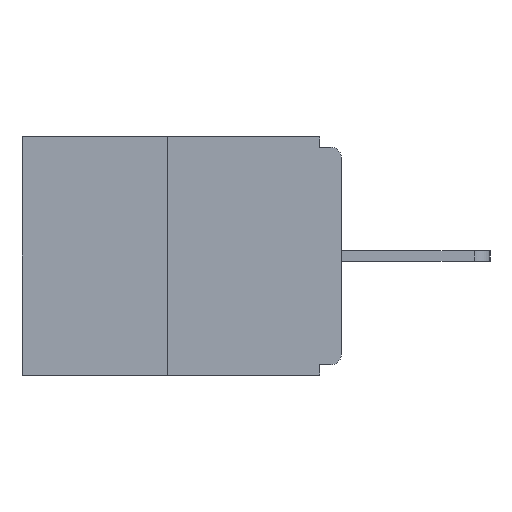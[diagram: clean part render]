
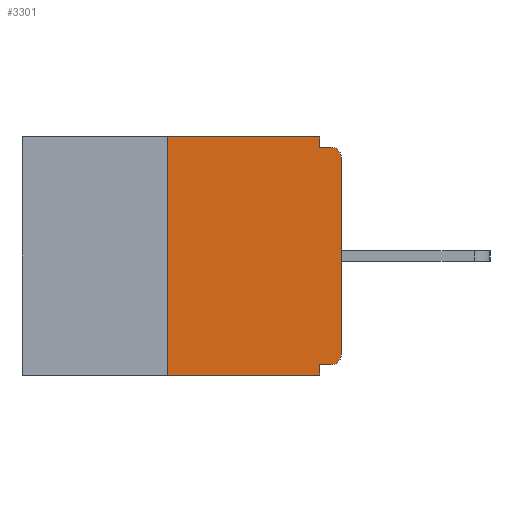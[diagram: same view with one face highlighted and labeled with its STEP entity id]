
A CAD part, left-side view. The second image highlights one B-rep face of the part: STEP entity #3301.
In plain terms, the highlighted planar face has unit normal (-1, 0, 0).
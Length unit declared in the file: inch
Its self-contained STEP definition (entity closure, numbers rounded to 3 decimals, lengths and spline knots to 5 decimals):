
#242 = CARTESIAN_POINT ( 'NONE',  ( 0., 0.031, -0.343 ) ) ;
#343 = CARTESIAN_POINT ( 'NONE',  ( 0., 0., -0.03 ) ) ;
#456 = VERTEX_POINT ( 'NONE', #1524 ) ;
#548 = VECTOR ( 'NONE', #8571, 39.37008 ) ;
#653 = DIRECTION ( 'NONE',  ( -1., 0., 0. ) ) ;
#758 = DIRECTION ( 'NONE',  ( -1., 0., 0. ) ) ;
#955 = LINE ( 'NONE', #3076, #10718 ) ;
#1160 = LINE ( 'NONE', #10264, #548 ) ;
#1182 = AXIS2_PLACEMENT_3D ( 'NONE', #12285, #2567, #3556 ) ;
#1368 = LINE ( 'NONE', #5953, #6409 ) ;
#1451 = CARTESIAN_POINT ( 'NONE',  ( 0., 0.46, -0.343 ) ) ;
#1524 = CARTESIAN_POINT ( 'NONE',  ( 0., 0.031, -0.328 ) ) ;
#1727 = DIRECTION ( 'NONE',  ( 0., 0., -1. ) ) ;
#2088 = VECTOR ( 'NONE', #8111, 39.37008 ) ;
#2567 = DIRECTION ( 'NONE',  ( 1., 0., 0. ) ) ;
#2926 = VECTOR ( 'NONE', #6526, 39.37008 ) ;
#3076 = CARTESIAN_POINT ( 'NONE',  ( 0., 0., -0.015 ) ) ;
#3214 = VERTEX_POINT ( 'NONE', #10161 ) ;
#3280 = EDGE_CURVE ( 'NONE', #8709, #8806, #3807, .T. ) ;
#3301 = ADVANCED_FACE ( 'NONE', ( #7441 ), #3514, .F. ) ;
#3380 = CARTESIAN_POINT ( 'NONE',  ( 0., 0.015, -0.015 ) ) ;
#3514 = PLANE ( 'NONE',  #1182 ) ;
#3556 = DIRECTION ( 'NONE',  ( 0., 0., -1. ) ) ;
#3696 = EDGE_CURVE ( 'NONE', #6570, #8709, #9564, .T. ) ;
#3751 = DIRECTION ( 'NONE',  ( 0., 0., 1. ) ) ;
#3774 = ORIENTED_EDGE ( 'NONE', *, *, #6194, .F. ) ;
#3807 = CIRCLE ( 'NONE', #4046, 0.015 ) ;
#3837 = ORIENTED_EDGE ( 'NONE', *, *, #9181, .F. ) ;
#4046 = AXIS2_PLACEMENT_3D ( 'NONE', #10285, #653, #10321 ) ;
#4461 = ORIENTED_EDGE ( 'NONE', *, *, #4955, .F. ) ;
#4955 = EDGE_CURVE ( 'NONE', #3214, #456, #11382, .T. ) ;
#5015 = CARTESIAN_POINT ( 'NONE',  ( 0., 0., -0.313 ) ) ;
#5085 = VERTEX_POINT ( 'NONE', #242 ) ;
#5657 = EDGE_LOOP ( 'NONE', ( #6913, #8763, #9135, #3837, #4461, #11863, #7188, #6697, #3774, #7486 ) ) ;
#5775 = DIRECTION ( 'NONE',  ( 0., 0., -1. ) ) ;
#5953 = CARTESIAN_POINT ( 'NONE',  ( 0., 0.031, 0. ) ) ;
#6194 = EDGE_CURVE ( 'NONE', #11292, #8806, #955, .T. ) ;
#6408 = CARTESIAN_POINT ( 'NONE',  ( 0., 0.031, -0.015 ) ) ;
#6409 = VECTOR ( 'NONE', #5775, 39.37008 ) ;
#6477 = CARTESIAN_POINT ( 'NONE',  ( 0., 0.015, -0.313 ) ) ;
#6526 = DIRECTION ( 'NONE',  ( 0., -1., 0. ) ) ;
#6527 = VECTOR ( 'NONE', #3751, 39.37008 ) ;
#6570 = VERTEX_POINT ( 'NONE', #5015 ) ;
#6575 = CARTESIAN_POINT ( 'NONE',  ( 0., 0.25, -0.343 ) ) ;
#6686 = EDGE_CURVE ( 'NONE', #8101, #7607, #10709, .T. ) ;
#6697 = ORIENTED_EDGE ( 'NONE', *, *, #3280, .T. ) ;
#6827 = DIRECTION ( 'NONE',  ( 0., 1., 0. ) ) ;
#6913 = ORIENTED_EDGE ( 'NONE', *, *, #6686, .F. ) ;
#7188 = ORIENTED_EDGE ( 'NONE', *, *, #3696, .T. ) ;
#7441 = FACE_OUTER_BOUND ( 'NONE', #5657, .T. ) ;
#7486 = ORIENTED_EDGE ( 'NONE', *, *, #7558, .F. ) ;
#7558 = EDGE_CURVE ( 'NONE', #7607, #11292, #1368, .T. ) ;
#7607 = VERTEX_POINT ( 'NONE', #10770 ) ;
#7707 = LINE ( 'NONE', #10428, #10005 ) ;
#8101 = VERTEX_POINT ( 'NONE', #12444 ) ;
#8111 = DIRECTION ( 'NONE',  ( 0., -1., 0. ) ) ;
#8223 = VERTEX_POINT ( 'NONE', #6575 ) ;
#8459 = CARTESIAN_POINT ( 'NONE',  ( 0., 0.46, 0. ) ) ;
#8571 = DIRECTION ( 'NONE',  ( 0., 0., -1. ) ) ;
#8709 = VERTEX_POINT ( 'NONE', #343 ) ;
#8763 = ORIENTED_EDGE ( 'NONE', *, *, #9262, .F. ) ;
#8806 = VERTEX_POINT ( 'NONE', #3380 ) ;
#8810 = VECTOR ( 'NONE', #6827, 39.37008 ) ;
#8951 = DIRECTION ( 'NONE',  ( 0., -1., 0. ) ) ;
#9135 = ORIENTED_EDGE ( 'NONE', *, *, #12295, .T. ) ;
#9181 = EDGE_CURVE ( 'NONE', #456, #5085, #1160, .T. ) ;
#9262 = EDGE_CURVE ( 'NONE', #8223, #8101, #7707, .T. ) ;
#9463 = EDGE_CURVE ( 'NONE', #3214, #6570, #11518, .T. ) ;
#9538 = CARTESIAN_POINT ( 'NONE',  ( 0., 0., 0. ) ) ;
#9564 = LINE ( 'NONE', #9538, #6527 ) ;
#9565 = DIRECTION ( 'NONE',  ( 0., 0., 1. ) ) ;
#9710 = LINE ( 'NONE', #1451, #2088 ) ;
#10005 = VECTOR ( 'NONE', #9565, 39.37008 ) ;
#10161 = CARTESIAN_POINT ( 'NONE',  ( 0., 0.015, -0.328 ) ) ;
#10264 = CARTESIAN_POINT ( 'NONE',  ( 0., 0.031, -0.343 ) ) ;
#10285 = CARTESIAN_POINT ( 'NONE',  ( 0., 0.015, -0.03 ) ) ;
#10321 = DIRECTION ( 'NONE',  ( 0., 0., -1. ) ) ;
#10428 = CARTESIAN_POINT ( 'NONE',  ( 0., 0.25, 0. ) ) ;
#10625 = CARTESIAN_POINT ( 'NONE',  ( 0., 0., -0.328 ) ) ;
#10709 = LINE ( 'NONE', #8459, #2926 ) ;
#10718 = VECTOR ( 'NONE', #8951, 39.37008 ) ;
#10770 = CARTESIAN_POINT ( 'NONE',  ( 0., 0.031, 0. ) ) ;
#11292 = VERTEX_POINT ( 'NONE', #6408 ) ;
#11382 = LINE ( 'NONE', #10625, #8810 ) ;
#11518 = CIRCLE ( 'NONE', #12257, 0.015 ) ;
#11863 = ORIENTED_EDGE ( 'NONE', *, *, #9463, .T. ) ;
#12257 = AXIS2_PLACEMENT_3D ( 'NONE', #6477, #758, #1727 ) ;
#12285 = CARTESIAN_POINT ( 'NONE',  ( 0., 0.46, 0. ) ) ;
#12295 = EDGE_CURVE ( 'NONE', #8223, #5085, #9710, .T. ) ;
#12444 = CARTESIAN_POINT ( 'NONE',  ( 0., 0.25, 0. ) ) ;
